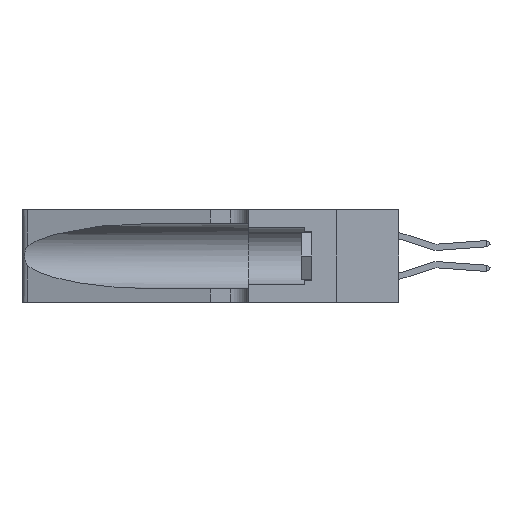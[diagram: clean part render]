
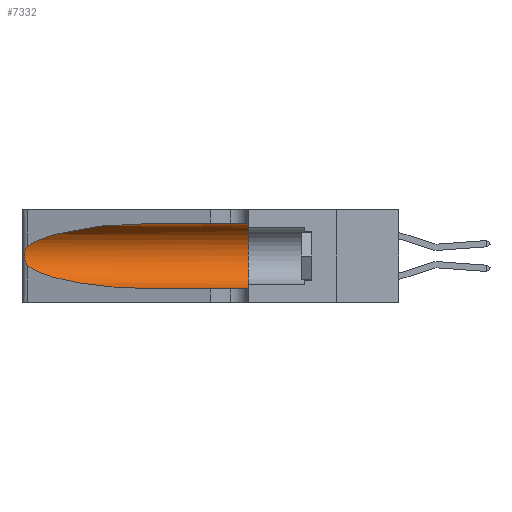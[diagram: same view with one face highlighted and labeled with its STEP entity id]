
A CAD part, left-side view. The second image highlights one B-rep face of the part: STEP entity #7332.
In plain terms, the highlighted cylindrical face has radius 3.308 mm (diameter 6.617 mm), a partial arc.
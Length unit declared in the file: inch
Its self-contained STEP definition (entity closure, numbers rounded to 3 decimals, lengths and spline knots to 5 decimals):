
#249 = CARTESIAN_POINT ( 'NONE',  ( 0.25487, 1.22718, 0.14631 ) ) ;
#612 = CARTESIAN_POINT ( 'NONE',  ( 0.25487, 1.22718, 0.14631 ) ) ;
#1598 = CARTESIAN_POINT ( 'NONE',  ( 0.1305, 0.35, 0.185 ) ) ;
#1667 = AXIS2_PLACEMENT_3D ( 'NONE', #1598, #20500, #11364 ) ;
#1724 =( BOUNDED_CURVE ( )  B_SPLINE_CURVE ( 3, ( #9960, #10357, #25861, #5833 ),
 .UNSPECIFIED., .F., .F. ) 
 B_SPLINE_CURVE_WITH_KNOTS ( ( 4, 4 ),
 ( 1.5708, 2.84003 ),
 .UNSPECIFIED. ) 
 CURVE ( )  GEOMETRIC_REPRESENTATION_ITEM ( )  RATIONAL_B_SPLINE_CURVE ( ( 1., 0.87, 0.87, 1. ) ) 
 REPRESENTATION_ITEM ( '' )  );
#2222 = CARTESIAN_POINT ( 'NONE',  ( 0.26018, 1.23835, 0.19895 ) ) ;
#2315 = CARTESIAN_POINT ( 'NONE',  ( 0.25487, 1.22718, 0.22369 ) ) ;
#2663 = VERTEX_POINT ( 'NONE', #16808 ) ;
#4494 = CARTESIAN_POINT ( 'NONE',  ( 0.25639, 1.23184, 0.21858 ) ) ;
#4894 = DIRECTION ( 'NONE',  ( 0., 0., -1. ) ) ;
#5035 = EDGE_CURVE ( 'NONE', #8001, #16757, #11393, .T. ) ;
#5833 = CARTESIAN_POINT ( 'NONE',  ( 0.25487, 1.22718, 0.22369 ) ) ;
#5854 = CARTESIAN_POINT ( 'NONE',  ( 0.1305, 0.72297, 0.05475 ) ) ;
#5998 = FACE_OUTER_BOUND ( 'NONE', #18364, .T. ) ;
#6664 = CARTESIAN_POINT ( 'NONE',  ( 0.25555, 1.22994, 0.2215 ) ) ;
#6863 = CARTESIAN_POINT ( 'NONE',  ( 0.26075, 1.23896, 0.178 ) ) ;
#7058 = ORIENTED_EDGE ( 'NONE', *, *, #20226, .T. ) ;
#7118 = LINE ( 'NONE', #10337, #17766 ) ;
#7332 = ADVANCED_FACE ( 'NONE', ( #5998 ), #9163, .F. ) ;
#7875 = EDGE_CURVE ( 'NONE', #16757, #2663, #10894, .T. ) ;
#8001 = VERTEX_POINT ( 'NONE', #28117 ) ;
#9031 = CARTESIAN_POINT ( 'NONE',  ( 0.26075, 1.23896, 0.19203 ) ) ;
#9163 = CYLINDRICAL_SURFACE ( 'NONE', #25428, 0.13025 ) ;
#9960 = CARTESIAN_POINT ( 'NONE',  ( 0.1305, 0.72297, 0.31525 ) ) ;
#9973 = VECTOR ( 'NONE', #22033, 39.37008 ) ;
#10337 = CARTESIAN_POINT ( 'NONE',  ( 0.1305, 1.61858, 0.05475 ) ) ;
#10357 = CARTESIAN_POINT ( 'NONE',  ( 0.18966, 0.96281, 0.31525 ) ) ;
#10454 = EDGE_CURVE ( 'NONE', #21710, #27296, #15710, .T. ) ;
#10894 = CIRCLE ( 'NONE', #1667, 0.13025 ) ;
#11303 = CARTESIAN_POINT ( 'NONE',  ( 0.25854, 1.2359, 0.20912 ) ) ;
#11364 = DIRECTION ( 'NONE',  ( 0., 0., 1. ) ) ;
#11393 = LINE ( 'NONE', #22324, #9973 ) ;
#11408 = CARTESIAN_POINT ( 'NONE',  ( 0.25789, 1.23486, 0.15765 ) ) ;
#13519 = ORIENTED_EDGE ( 'NONE', *, *, #5035, .F. ) ;
#13688 = CARTESIAN_POINT ( 'NONE',  ( 0.25639, 1.23186, 0.15144 ) ) ;
#14092 = CARTESIAN_POINT ( 'NONE',  ( 0.18966, 0.96281, 0.05475 ) ) ;
#14841 = CARTESIAN_POINT ( 'NONE',  ( 0.1305, 0.35, 0.31525 ) ) ;
#15189 = EDGE_CURVE ( 'NONE', #8001, #16963, #1724, .T. ) ;
#15388 = ORIENTED_EDGE ( 'NONE', *, *, #7875, .F. ) ;
#15425 = CARTESIAN_POINT ( 'NONE',  ( 0.1305, 1.61858, 0.185 ) ) ;
#15710 =( BOUNDED_CURVE ( )  B_SPLINE_CURVE ( 3, ( #18568, #27630, #14092, #23211 ),
 .UNSPECIFIED., .F., .F. ) 
 B_SPLINE_CURVE_WITH_KNOTS ( ( 4, 4 ),
 ( 3.44316, 4.71239 ),
 .UNSPECIFIED. ) 
 CURVE ( )  GEOMETRIC_REPRESENTATION_ITEM ( )  RATIONAL_B_SPLINE_CURVE ( ( 1., 0.87, 0.87, 1. ) ) 
 REPRESENTATION_ITEM ( '' )  );
#16757 = VERTEX_POINT ( 'NONE', #14841 ) ;
#16808 = CARTESIAN_POINT ( 'NONE',  ( 0.1305, 0.35, 0.05475 ) ) ;
#16963 = VERTEX_POINT ( 'NONE', #2315 ) ;
#17766 = VECTOR ( 'NONE', #19375, 39.37008 ) ;
#18364 = EDGE_LOOP ( 'NONE', ( #26197, #7058, #19266, #26584, #15388, #13519 ) ) ;
#18568 = CARTESIAN_POINT ( 'NONE',  ( 0.25487, 1.22718, 0.14631 ) ) ;
#19266 = ORIENTED_EDGE ( 'NONE', *, *, #10454, .T. ) ;
#19375 = DIRECTION ( 'NONE',  ( 0., -1., 0. ) ) ;
#19962 = EDGE_CURVE ( 'NONE', #27296, #2663, #7118, .T. ) ;
#19967 = DIRECTION ( 'NONE',  ( 0., -1., 0. ) ) ;
#20226 = EDGE_CURVE ( 'NONE', #16963, #21710, #23697, .T. ) ;
#20247 = CARTESIAN_POINT ( 'NONE',  ( 0.25487, 1.22718, 0.22369 ) ) ;
#20500 = DIRECTION ( 'NONE',  ( 0., 1., 0. ) ) ;
#21710 = VERTEX_POINT ( 'NONE', #249 ) ;
#22033 = DIRECTION ( 'NONE',  ( 0., -1., 0. ) ) ;
#22324 = CARTESIAN_POINT ( 'NONE',  ( 0.1305, 1.61858, 0.31525 ) ) ;
#22730 = CARTESIAN_POINT ( 'NONE',  ( 0.26017, 1.23833, 0.17102 ) ) ;
#23211 = CARTESIAN_POINT ( 'NONE',  ( 0.1305, 0.72297, 0.05475 ) ) ;
#23697 = B_SPLINE_CURVE_WITH_KNOTS ( 'NONE', 3,
 ( #20247, #6664, #4494, #24814, #11303, #2222, #9031, #6863, #22730, #25010, #11408, #13688, #27608, #612 ),
 .UNSPECIFIED., .F., .F.,
 ( 4, 2, 2, 2, 2, 2, 4 ),
 ( 0., 0.00027, 0.00053, 0.00107, 0.0016, 0.00187, 0.00214 ),
 .UNSPECIFIED. ) ;
#24814 = CARTESIAN_POINT ( 'NONE',  ( 0.25787, 1.23484, 0.2124 ) ) ;
#25010 = CARTESIAN_POINT ( 'NONE',  ( 0.25856, 1.23593, 0.16098 ) ) ;
#25428 = AXIS2_PLACEMENT_3D ( 'NONE', #15425, #19967, #4894 ) ;
#25861 = CARTESIAN_POINT ( 'NONE',  ( 0.2373, 1.15595, 0.28018 ) ) ;
#26197 = ORIENTED_EDGE ( 'NONE', *, *, #15189, .T. ) ;
#26584 = ORIENTED_EDGE ( 'NONE', *, *, #19962, .T. ) ;
#27296 = VERTEX_POINT ( 'NONE', #5854 ) ;
#27608 = CARTESIAN_POINT ( 'NONE',  ( 0.25555, 1.22993, 0.14849 ) ) ;
#27630 = CARTESIAN_POINT ( 'NONE',  ( 0.2373, 1.15595, 0.08982 ) ) ;
#28117 = CARTESIAN_POINT ( 'NONE',  ( 0.1305, 0.72297, 0.31525 ) ) ;
